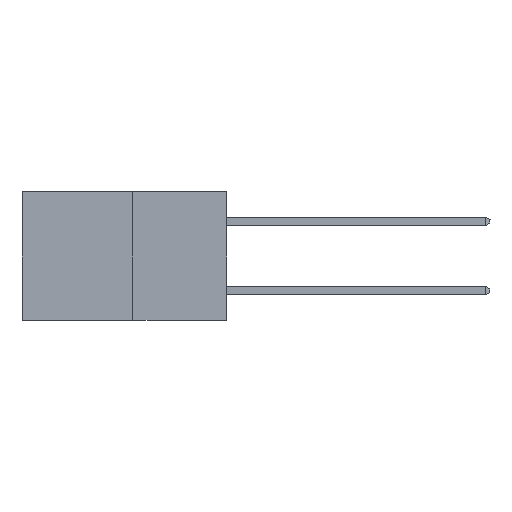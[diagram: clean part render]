
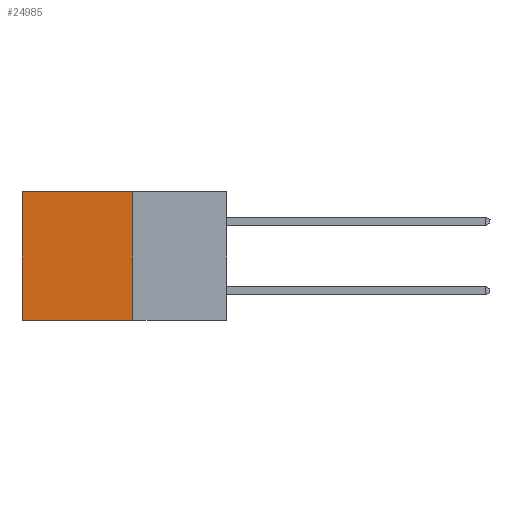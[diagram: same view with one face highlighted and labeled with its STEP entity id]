
A CAD part, left-side view. The second image highlights one B-rep face of the part: STEP entity #24985.
In plain terms, the highlighted planar face has unit normal (-1, 0, 0).
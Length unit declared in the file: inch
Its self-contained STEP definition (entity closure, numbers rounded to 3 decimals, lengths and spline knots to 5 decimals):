
#40 = ORIENTED_EDGE ( 'NONE', *, *, #29283, .T. ) ;
#918 = FACE_OUTER_BOUND ( 'NONE', #16500, .T. ) ;
#2957 = PLANE ( 'NONE',  #19476 ) ;
#4058 = CARTESIAN_POINT ( 'NONE',  ( 0.277, 0.59, -0.37 ) ) ;
#4218 = VECTOR ( 'NONE', #11000, 39.37008 ) ;
#6113 = EDGE_CURVE ( 'NONE', #25252, #7965, #9681, .T. ) ;
#6676 = ORIENTED_EDGE ( 'NONE', *, *, #20390, .F. ) ;
#7965 = VERTEX_POINT ( 'NONE', #4058 ) ;
#8217 = CARTESIAN_POINT ( 'NONE',  ( 0.277, 0.59, -0.37 ) ) ;
#8592 = DIRECTION ( 'NONE',  ( 1., 0., 0. ) ) ;
#9261 = VECTOR ( 'NONE', #16451, 39.37008 ) ;
#9681 = LINE ( 'NONE', #29408, #17035 ) ;
#9968 = DIRECTION ( 'NONE',  ( 0., 1., 0. ) ) ;
#11000 = DIRECTION ( 'NONE',  ( 0., 0., -1. ) ) ;
#12651 = DIRECTION ( 'NONE',  ( 0., 1., 0. ) ) ;
#12812 = CARTESIAN_POINT ( 'NONE',  ( 0.277, 0.59, 0. ) ) ;
#13677 = CARTESIAN_POINT ( 'NONE',  ( 0.277, 0.27, -0.37 ) ) ;
#14958 = ORIENTED_EDGE ( 'NONE', *, *, #6113, .F. ) ;
#16451 = DIRECTION ( 'NONE',  ( 0., 0., -1. ) ) ;
#16500 = EDGE_LOOP ( 'NONE', ( #26690, #14958, #6676, #40 ) ) ;
#16813 = CARTESIAN_POINT ( 'NONE',  ( 0.277, 0.27, -0.37 ) ) ;
#17035 = VECTOR ( 'NONE', #9968, 39.37008 ) ;
#17605 = LINE ( 'NONE', #18211, #24959 ) ;
#18211 = CARTESIAN_POINT ( 'NONE',  ( 0.277, 0.27, 0. ) ) ;
#19476 = AXIS2_PLACEMENT_3D ( 'NONE', #16813, #8592, #27962 ) ;
#20390 = EDGE_CURVE ( 'NONE', #21085, #25252, #31318, .T. ) ;
#20852 = VERTEX_POINT ( 'NONE', #12812 ) ;
#21085 = VERTEX_POINT ( 'NONE', #35606 ) ;
#23438 = EDGE_CURVE ( 'NONE', #20852, #7965, #26352, .T. ) ;
#24959 = VECTOR ( 'NONE', #12651, 39.37008 ) ;
#24985 = ADVANCED_FACE ( 'NONE', ( #918 ), #2957, .F. ) ;
#25252 = VERTEX_POINT ( 'NONE', #34432 ) ;
#26352 = LINE ( 'NONE', #8217, #4218 ) ;
#26690 = ORIENTED_EDGE ( 'NONE', *, *, #23438, .T. ) ;
#27962 = DIRECTION ( 'NONE',  ( 0., 0., -1. ) ) ;
#29283 = EDGE_CURVE ( 'NONE', #21085, #20852, #17605, .T. ) ;
#29408 = CARTESIAN_POINT ( 'NONE',  ( 0.277, 0.27, -0.37 ) ) ;
#31318 = LINE ( 'NONE', #13677, #9261 ) ;
#34432 = CARTESIAN_POINT ( 'NONE',  ( 0.277, 0.27, -0.37 ) ) ;
#35606 = CARTESIAN_POINT ( 'NONE',  ( 0.277, 0.27, 0. ) ) ;
